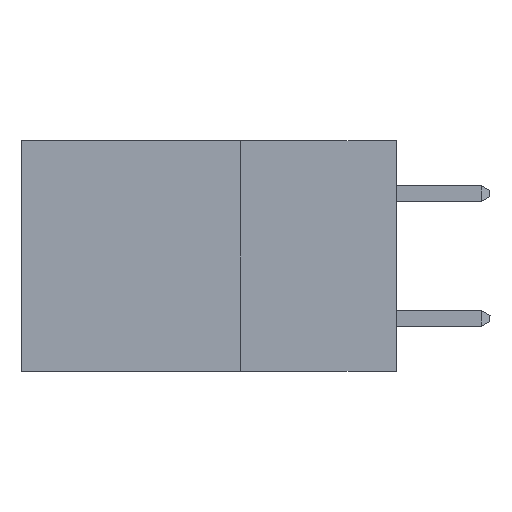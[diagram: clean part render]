
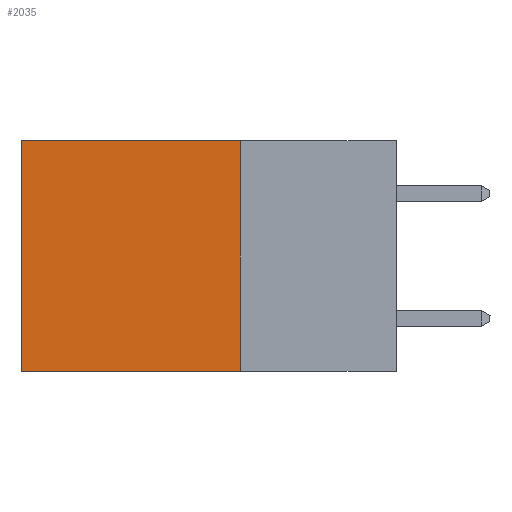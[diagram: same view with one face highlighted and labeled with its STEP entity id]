
A CAD part, left-side view. The second image highlights one B-rep face of the part: STEP entity #2035.
In plain terms, the highlighted planar face has unit normal (-1, 0, 0).
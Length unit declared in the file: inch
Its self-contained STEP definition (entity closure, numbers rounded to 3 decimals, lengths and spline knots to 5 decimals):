
#574 = LINE ( 'NONE', #1022, #6393 ) ;
#980 = DIRECTION ( 'NONE',  ( 0., 1., 0. ) ) ;
#1022 = CARTESIAN_POINT ( 'NONE',  ( 0.2615, 0.25, 0. ) ) ;
#1244 = CARTESIAN_POINT ( 'NONE',  ( 0.2615, 0.25, 0. ) ) ;
#1396 = ORIENTED_EDGE ( 'NONE', *, *, #7120, .F. ) ;
#1551 = VERTEX_POINT ( 'NONE', #6919 ) ;
#1602 = CARTESIAN_POINT ( 'NONE',  ( 0.2615, 0.25, -0.37 ) ) ;
#2035 = ADVANCED_FACE ( 'NONE', ( #12118 ), #13802, .F. ) ;
#2232 = DIRECTION ( 'NONE',  ( 0., 0., -1. ) ) ;
#2386 = CARTESIAN_POINT ( 'NONE',  ( 0.2615, 0.6, -0.37 ) ) ;
#4034 = VECTOR ( 'NONE', #14097, 39.37008 ) ;
#4326 = EDGE_CURVE ( 'NONE', #9988, #11271, #14473, .T. ) ;
#4656 = VECTOR ( 'NONE', #2232, 39.37008 ) ;
#5759 = DIRECTION ( 'NONE',  ( 0., 1., 0. ) ) ;
#6393 = VECTOR ( 'NONE', #980, 39.37008 ) ;
#6584 = CARTESIAN_POINT ( 'NONE',  ( 0.2615, 0.25, -0.37 ) ) ;
#6802 = CARTESIAN_POINT ( 'NONE',  ( 0.2615, 0.6, -0.37 ) ) ;
#6919 = CARTESIAN_POINT ( 'NONE',  ( 0.2615, 0.6, 0. ) ) ;
#7120 = EDGE_CURVE ( 'NONE', #7203, #9988, #10613, .T. ) ;
#7203 = VERTEX_POINT ( 'NONE', #1244 ) ;
#8593 = AXIS2_PLACEMENT_3D ( 'NONE', #13434, #13203, #13422 ) ;
#9988 = VERTEX_POINT ( 'NONE', #1602 ) ;
#10588 = ORIENTED_EDGE ( 'NONE', *, *, #11879, .T. ) ;
#10613 = LINE ( 'NONE', #14225, #4034 ) ;
#11174 = VECTOR ( 'NONE', #5759, 39.37008 ) ;
#11271 = VERTEX_POINT ( 'NONE', #6802 ) ;
#11636 = EDGE_LOOP ( 'NONE', ( #10588, #14251, #1396, #12718 ) ) ;
#11879 = EDGE_CURVE ( 'NONE', #1551, #11271, #13798, .T. ) ;
#12101 = EDGE_CURVE ( 'NONE', #7203, #1551, #574, .T. ) ;
#12118 = FACE_OUTER_BOUND ( 'NONE', #11636, .T. ) ;
#12718 = ORIENTED_EDGE ( 'NONE', *, *, #12101, .T. ) ;
#13203 = DIRECTION ( 'NONE',  ( 1., 0., 0. ) ) ;
#13422 = DIRECTION ( 'NONE',  ( 0., 0., -1. ) ) ;
#13434 = CARTESIAN_POINT ( 'NONE',  ( 0.2615, 0.25, -0.37 ) ) ;
#13798 = LINE ( 'NONE', #2386, #4656 ) ;
#13802 = PLANE ( 'NONE',  #8593 ) ;
#14097 = DIRECTION ( 'NONE',  ( 0., 0., -1. ) ) ;
#14225 = CARTESIAN_POINT ( 'NONE',  ( 0.2615, 0.25, -0.37 ) ) ;
#14251 = ORIENTED_EDGE ( 'NONE', *, *, #4326, .F. ) ;
#14473 = LINE ( 'NONE', #6584, #11174 ) ;
